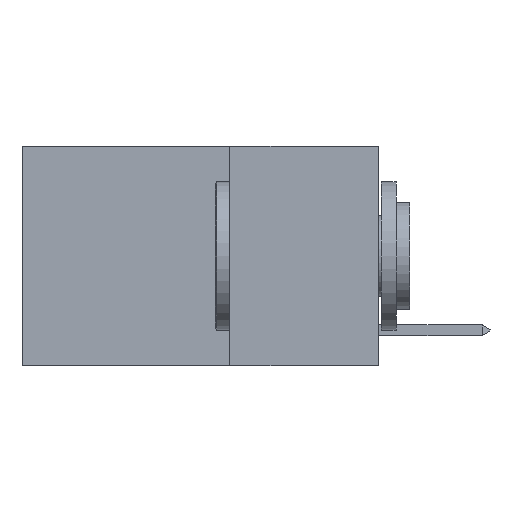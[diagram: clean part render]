
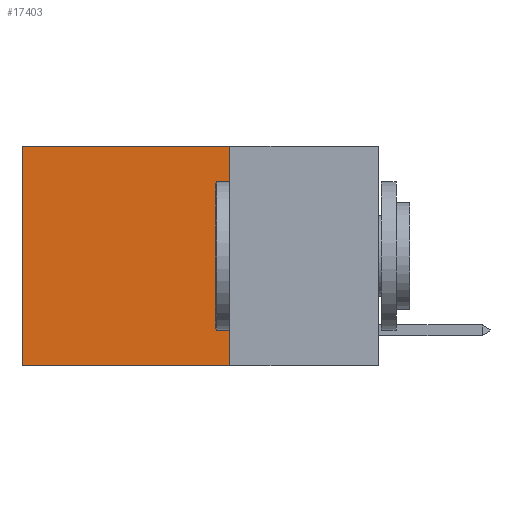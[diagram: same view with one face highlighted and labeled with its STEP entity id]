
A CAD part, left-side view. The second image highlights one B-rep face of the part: STEP entity #17403.
In plain terms, the highlighted planar face has unit normal (-1, 0, 0).
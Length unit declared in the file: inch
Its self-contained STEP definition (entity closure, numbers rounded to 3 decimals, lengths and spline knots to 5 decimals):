
#312 = VERTEX_POINT ( 'NONE', #9668 ) ;
#908 = ORIENTED_EDGE ( 'NONE', *, *, #15419, .T. ) ;
#964 = DIRECTION ( 'NONE',  ( 1., 0., 0. ) ) ;
#1436 = ORIENTED_EDGE ( 'NONE', *, *, #9166, .T. ) ;
#2426 = EDGE_CURVE ( 'NONE', #3588, #312, #6291, .T. ) ;
#3588 = VERTEX_POINT ( 'NONE', #22251 ) ;
#3898 = VERTEX_POINT ( 'NONE', #6750 ) ;
#4323 = ORIENTED_EDGE ( 'NONE', *, *, #5452, .F. ) ;
#4973 = CARTESIAN_POINT ( 'NONE',  ( 0.2625, 0.25, 0. ) ) ;
#5033 = AXIS2_PLACEMENT_3D ( 'NONE', #19883, #964, #9398 ) ;
#5452 = EDGE_CURVE ( 'NONE', #312, #3898, #8129, .T. ) ;
#5836 = VECTOR ( 'NONE', #25367, 39.37008 ) ;
#6291 = LINE ( 'NONE', #19169, #5836 ) ;
#6750 = CARTESIAN_POINT ( 'NONE',  ( 0.2625, 0.6, -0.37 ) ) ;
#8129 = LINE ( 'NONE', #10481, #24369 ) ;
#9166 = EDGE_CURVE ( 'NONE', #13250, #3898, #19644, .T. ) ;
#9398 = DIRECTION ( 'NONE',  ( 0., 0., -1. ) ) ;
#9668 = CARTESIAN_POINT ( 'NONE',  ( 0.2625, 0.25, -0.37 ) ) ;
#10481 = CARTESIAN_POINT ( 'NONE',  ( 0.2625, 0.25, -0.37 ) ) ;
#11228 = LINE ( 'NONE', #4973, #19530 ) ;
#11359 = DIRECTION ( 'NONE',  ( 0., 0., -1. ) ) ;
#11363 = DIRECTION ( 'NONE',  ( 0., 1., 0. ) ) ;
#11463 = PLANE ( 'NONE',  #5033 ) ;
#11750 = FACE_OUTER_BOUND ( 'NONE', #16308, .T. ) ;
#13158 = CARTESIAN_POINT ( 'NONE',  ( 0.2625, 0.6, 0. ) ) ;
#13250 = VERTEX_POINT ( 'NONE', #14453 ) ;
#13864 = ORIENTED_EDGE ( 'NONE', *, *, #2426, .F. ) ;
#14453 = CARTESIAN_POINT ( 'NONE',  ( 0.2625, 0.6, 0. ) ) ;
#14850 = VECTOR ( 'NONE', #11359, 39.37008 ) ;
#15419 = EDGE_CURVE ( 'NONE', #3588, #13250, #11228, .T. ) ;
#16308 = EDGE_LOOP ( 'NONE', ( #1436, #4323, #13864, #908 ) ) ;
#17403 = ADVANCED_FACE ( 'NONE', ( #11750 ), #11463, .F. ) ;
#19169 = CARTESIAN_POINT ( 'NONE',  ( 0.2625, 0.25, 0. ) ) ;
#19530 = VECTOR ( 'NONE', #11363, 39.37008 ) ;
#19644 = LINE ( 'NONE', #13158, #14850 ) ;
#19883 = CARTESIAN_POINT ( 'NONE',  ( 0.2625, 0.25, 0. ) ) ;
#22251 = CARTESIAN_POINT ( 'NONE',  ( 0.2625, 0.25, 0. ) ) ;
#23024 = DIRECTION ( 'NONE',  ( 0., 1., 0. ) ) ;
#24369 = VECTOR ( 'NONE', #23024, 39.37008 ) ;
#25367 = DIRECTION ( 'NONE',  ( 0., 0., -1. ) ) ;
